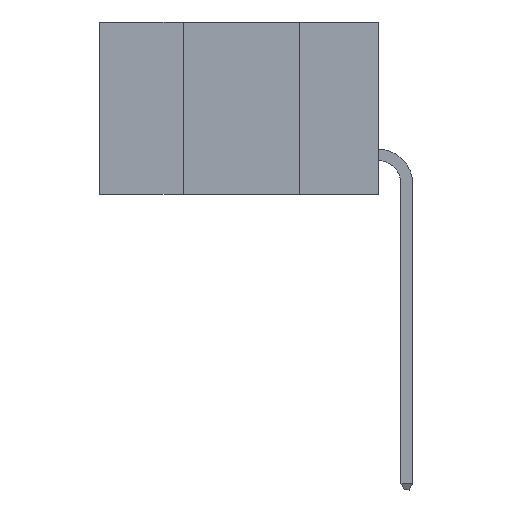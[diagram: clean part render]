
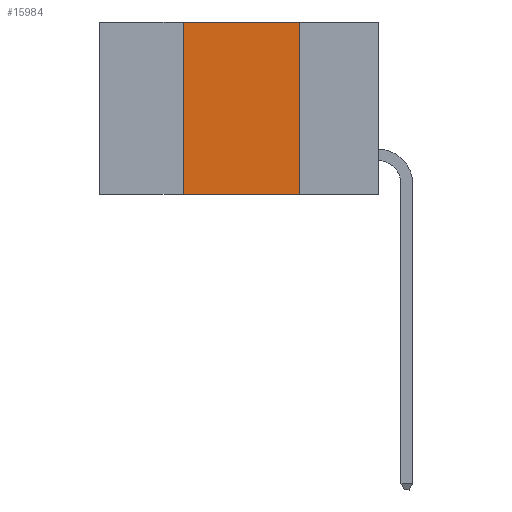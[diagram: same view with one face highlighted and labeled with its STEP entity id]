
A CAD part, left-side view. The second image highlights one B-rep face of the part: STEP entity #15984.
In plain terms, the highlighted planar face has unit normal (-1, 0, 0).
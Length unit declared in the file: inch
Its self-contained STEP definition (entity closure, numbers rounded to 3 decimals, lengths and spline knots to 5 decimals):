
#274 = LINE ( 'NONE', #7862, #2716 ) ;
#430 = PLANE ( 'NONE',  #27294 ) ;
#507 = VECTOR ( 'NONE', #26992, 39.37008 ) ;
#1525 = CARTESIAN_POINT ( 'NONE',  ( 0., 0.42, 0. ) ) ;
#1528 = ORIENTED_EDGE ( 'NONE', *, *, #28179, .F. ) ;
#2386 = DIRECTION ( 'NONE',  ( 0., 0., -1. ) ) ;
#2716 = VECTOR ( 'NONE', #12314, 39.37008 ) ;
#3275 = ORIENTED_EDGE ( 'NONE', *, *, #18151, .F. ) ;
#3689 = EDGE_CURVE ( 'NONE', #26735, #21836, #274, .T. ) ;
#3705 = VERTEX_POINT ( 'NONE', #19536 ) ;
#4911 = CARTESIAN_POINT ( 'NONE',  ( 0., 0.17, 0. ) ) ;
#6715 = LINE ( 'NONE', #6785, #17891 ) ;
#6785 = CARTESIAN_POINT ( 'NONE',  ( 0., 0.6, 0. ) ) ;
#7862 = CARTESIAN_POINT ( 'NONE',  ( 0., 0.6, -0.37 ) ) ;
#9179 = ORIENTED_EDGE ( 'NONE', *, *, #3689, .T. ) ;
#9243 = DIRECTION ( 'NONE',  ( 0., 0., -1. ) ) ;
#9947 = VECTOR ( 'NONE', #9243, 39.37008 ) ;
#10326 = LINE ( 'NONE', #22677, #507 ) ;
#12314 = DIRECTION ( 'NONE',  ( 0., -1., 0. ) ) ;
#13512 = CARTESIAN_POINT ( 'NONE',  ( 0., 0.6, 0. ) ) ;
#13594 = EDGE_CURVE ( 'NONE', #3705, #21836, #22152, .T. ) ;
#15984 = ADVANCED_FACE ( 'NONE', ( #20971 ), #430, .F. ) ;
#16834 = CARTESIAN_POINT ( 'NONE',  ( 0., 0.17, -0.37 ) ) ;
#17891 = VECTOR ( 'NONE', #26715, 39.37008 ) ;
#18151 = EDGE_CURVE ( 'NONE', #22162, #3705, #6715, .T. ) ;
#19536 = CARTESIAN_POINT ( 'NONE',  ( 0., 0.17, 0. ) ) ;
#20971 = FACE_OUTER_BOUND ( 'NONE', #23040, .T. ) ;
#21225 = ORIENTED_EDGE ( 'NONE', *, *, #13594, .F. ) ;
#21836 = VERTEX_POINT ( 'NONE', #16834 ) ;
#22152 = LINE ( 'NONE', #4911, #9947 ) ;
#22162 = VERTEX_POINT ( 'NONE', #1525 ) ;
#22623 = DIRECTION ( 'NONE',  ( 1., 0., 0. ) ) ;
#22677 = CARTESIAN_POINT ( 'NONE',  ( 0., 0.42, 0. ) ) ;
#23040 = EDGE_LOOP ( 'NONE', ( #21225, #3275, #1528, #9179 ) ) ;
#26715 = DIRECTION ( 'NONE',  ( 0., -1., 0. ) ) ;
#26735 = VERTEX_POINT ( 'NONE', #27174 ) ;
#26992 = DIRECTION ( 'NONE',  ( 0., 0., 1. ) ) ;
#27174 = CARTESIAN_POINT ( 'NONE',  ( 0., 0.42, -0.37 ) ) ;
#27294 = AXIS2_PLACEMENT_3D ( 'NONE', #13512, #22623, #2386 ) ;
#28179 = EDGE_CURVE ( 'NONE', #26735, #22162, #10326, .T. ) ;
